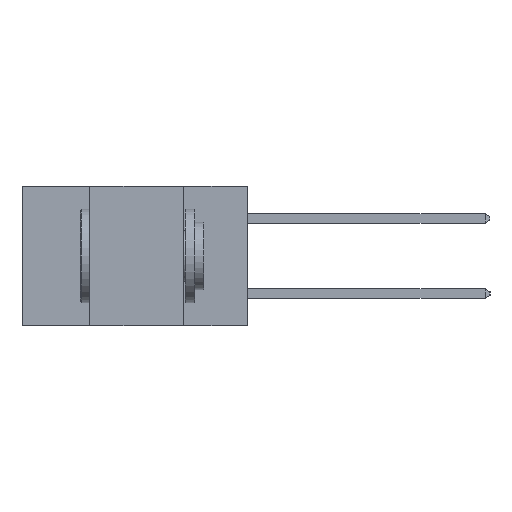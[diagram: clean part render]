
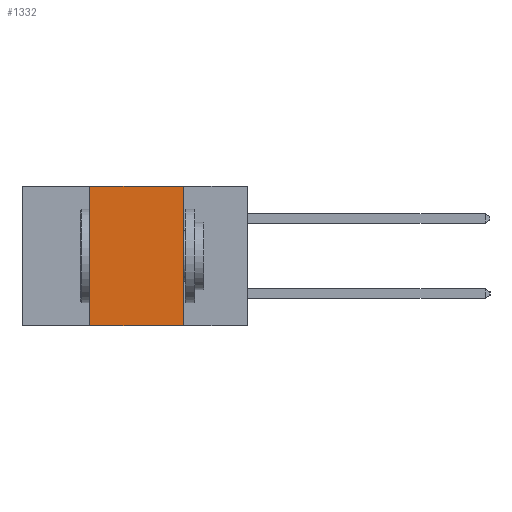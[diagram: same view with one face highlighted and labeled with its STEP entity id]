
A CAD part, left-side view. The second image highlights one B-rep face of the part: STEP entity #1332.
In plain terms, the highlighted planar face has unit normal (-1, 0, 0).
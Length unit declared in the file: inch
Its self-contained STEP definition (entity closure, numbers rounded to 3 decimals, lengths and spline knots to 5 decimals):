
#135 = LINE ( 'NONE', #5842, #4053 ) ;
#195 = CARTESIAN_POINT ( 'NONE',  ( 0., 0.42, -0.37 ) ) ;
#252 = VECTOR ( 'NONE', #7086, 39.37008 ) ;
#259 = EDGE_CURVE ( 'NONE', #5400, #6821, #135, .T. ) ;
#401 = CARTESIAN_POINT ( 'NONE',  ( 0., 0.17, 0. ) ) ;
#492 = LINE ( 'NONE', #2383, #252 ) ;
#613 = CARTESIAN_POINT ( 'NONE',  ( 0., 0.17, -0.37 ) ) ;
#633 = DIRECTION ( 'NONE',  ( 0., -1., 0. ) ) ;
#655 = CARTESIAN_POINT ( 'NONE',  ( 0., 0.6, 0. ) ) ;
#960 = EDGE_CURVE ( 'NONE', #5400, #1396, #492, .T. ) ;
#1332 = ADVANCED_FACE ( 'NONE', ( #1473 ), #4283, .F. ) ;
#1396 = VERTEX_POINT ( 'NONE', #8557 ) ;
#1473 = FACE_OUTER_BOUND ( 'NONE', #2553, .T. ) ;
#1911 = ORIENTED_EDGE ( 'NONE', *, *, #259, .F. ) ;
#2086 = VECTOR ( 'NONE', #633, 39.37008 ) ;
#2165 = ORIENTED_EDGE ( 'NONE', *, *, #960, .T. ) ;
#2343 = VECTOR ( 'NONE', #6555, 39.37008 ) ;
#2383 = CARTESIAN_POINT ( 'NONE',  ( 0., 0.6, -0.37 ) ) ;
#2553 = EDGE_LOOP ( 'NONE', ( #8771, #7236, #1911, #2165 ) ) ;
#4053 = VECTOR ( 'NONE', #5763, 39.37008 ) ;
#4067 = CARTESIAN_POINT ( 'NONE',  ( 0., 0.6, 0. ) ) ;
#4170 = AXIS2_PLACEMENT_3D ( 'NONE', #4067, #5010, #4975 ) ;
#4283 = PLANE ( 'NONE',  #4170 ) ;
#4975 = DIRECTION ( 'NONE',  ( 0., 0., -1. ) ) ;
#5010 = DIRECTION ( 'NONE',  ( 1., 0., 0. ) ) ;
#5400 = VERTEX_POINT ( 'NONE', #195 ) ;
#5763 = DIRECTION ( 'NONE',  ( 0., 0., 1. ) ) ;
#5842 = CARTESIAN_POINT ( 'NONE',  ( 0., 0.42, -0.37 ) ) ;
#6350 = EDGE_CURVE ( 'NONE', #6821, #6790, #6654, .T. ) ;
#6555 = DIRECTION ( 'NONE',  ( 0., 0., -1. ) ) ;
#6654 = LINE ( 'NONE', #655, #2086 ) ;
#6781 = EDGE_CURVE ( 'NONE', #6790, #1396, #8000, .T. ) ;
#6790 = VERTEX_POINT ( 'NONE', #401 ) ;
#6821 = VERTEX_POINT ( 'NONE', #7937 ) ;
#7086 = DIRECTION ( 'NONE',  ( 0., -1., 0. ) ) ;
#7236 = ORIENTED_EDGE ( 'NONE', *, *, #6350, .F. ) ;
#7937 = CARTESIAN_POINT ( 'NONE',  ( 0., 0.42, 0. ) ) ;
#8000 = LINE ( 'NONE', #613, #2343 ) ;
#8557 = CARTESIAN_POINT ( 'NONE',  ( 0., 0.17, -0.37 ) ) ;
#8771 = ORIENTED_EDGE ( 'NONE', *, *, #6781, .F. ) ;
